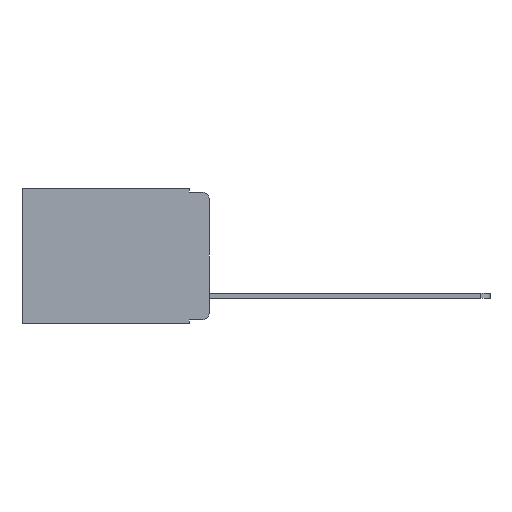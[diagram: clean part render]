
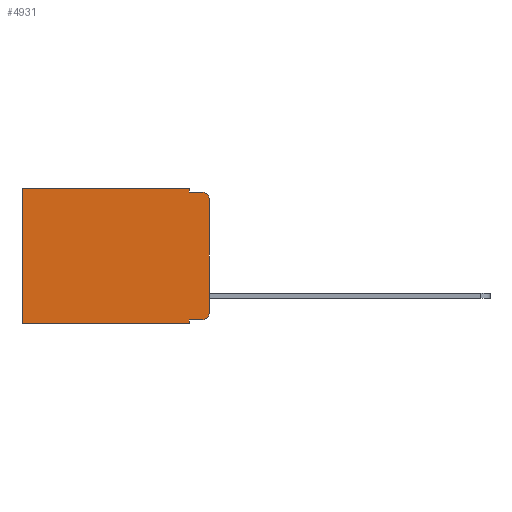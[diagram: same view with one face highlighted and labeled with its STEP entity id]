
A CAD part, left-side view. The second image highlights one B-rep face of the part: STEP entity #4931.
In plain terms, the highlighted planar face has unit normal (-1, 0, 0).
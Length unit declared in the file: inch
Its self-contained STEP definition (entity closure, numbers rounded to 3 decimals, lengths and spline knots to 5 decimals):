
#143 = CARTESIAN_POINT ( 'NONE',  ( 0.298, 0.051, 0. ) ) ;
#381 = DIRECTION ( 'NONE',  ( 0., 1., 0. ) ) ;
#595 = VECTOR ( 'NONE', #5572, 39.37008 ) ;
#621 = CARTESIAN_POINT ( 'NONE',  ( 0.298, 0.473, 0. ) ) ;
#640 = CARTESIAN_POINT ( 'NONE',  ( 0.298, 0.473, 0. ) ) ;
#706 = VERTEX_POINT ( 'NONE', #640 ) ;
#814 = ORIENTED_EDGE ( 'NONE', *, *, #1271, .F. ) ;
#954 = LINE ( 'NONE', #12647, #11044 ) ;
#975 = CARTESIAN_POINT ( 'NONE',  ( 0.298, 0.051, -0.343 ) ) ;
#1271 = EDGE_CURVE ( 'NONE', #1535, #10367, #11282, .T. ) ;
#1535 = VERTEX_POINT ( 'NONE', #975 ) ;
#2124 = LINE ( 'NONE', #621, #5305 ) ;
#2425 = FACE_OUTER_BOUND ( 'NONE', #9493, .T. ) ;
#2588 = ORIENTED_EDGE ( 'NONE', *, *, #4125, .F. ) ;
#2693 = DIRECTION ( 'NONE',  ( -1., 0., 0. ) ) ;
#2719 = VERTEX_POINT ( 'NONE', #5087 ) ;
#2850 = VERTEX_POINT ( 'NONE', #7768 ) ;
#3081 = VERTEX_POINT ( 'NONE', #11312 ) ;
#3576 = DIRECTION ( 'NONE',  ( -1., 0., 0. ) ) ;
#3596 = LINE ( 'NONE', #143, #11508 ) ;
#3645 = CARTESIAN_POINT ( 'NONE',  ( 0.298, 0.473, -0.343 ) ) ;
#3859 = EDGE_CURVE ( 'NONE', #11852, #1535, #12312, .T. ) ;
#3993 = VERTEX_POINT ( 'NONE', #8887 ) ;
#4125 = EDGE_CURVE ( 'NONE', #2850, #7974, #3596, .T. ) ;
#4300 = ORIENTED_EDGE ( 'NONE', *, *, #10126, .T. ) ;
#4311 = EDGE_CURVE ( 'NONE', #11852, #3081, #11987, .T. ) ;
#4498 = ORIENTED_EDGE ( 'NONE', *, *, #12675, .F. ) ;
#4522 = CIRCLE ( 'NONE', #8529, 0.02 ) ;
#4931 = ADVANCED_FACE ( 'NONE', ( #2425 ), #10984, .F. ) ;
#5087 = CARTESIAN_POINT ( 'NONE',  ( 0.298, 0.02, -0.01 ) ) ;
#5145 = DIRECTION ( 'NONE',  ( 1., 0., 0. ) ) ;
#5178 = CARTESIAN_POINT ( 'NONE',  ( 0.298, 0.02, -0.03 ) ) ;
#5304 = ORIENTED_EDGE ( 'NONE', *, *, #4311, .T. ) ;
#5305 = VECTOR ( 'NONE', #8052, 39.37008 ) ;
#5371 = AXIS2_PLACEMENT_3D ( 'NONE', #5178, #3576, #7369 ) ;
#5572 = DIRECTION ( 'NONE',  ( 0., -1., 0. ) ) ;
#5716 = CARTESIAN_POINT ( 'NONE',  ( 0.298, 0., -0.343 ) ) ;
#6243 = CARTESIAN_POINT ( 'NONE',  ( 0.298, 0.051, -0.333 ) ) ;
#6254 = AXIS2_PLACEMENT_3D ( 'NONE', #12766, #5145, #7292 ) ;
#6681 = VECTOR ( 'NONE', #381, 39.37008 ) ;
#6712 = EDGE_CURVE ( 'NONE', #10533, #2719, #10645, .T. ) ;
#6837 = ORIENTED_EDGE ( 'NONE', *, *, #7906, .T. ) ;
#6873 = CARTESIAN_POINT ( 'NONE',  ( 0.298, 0.051, -0.333 ) ) ;
#7198 = CARTESIAN_POINT ( 'NONE',  ( 0.298, 0., -0.03 ) ) ;
#7292 = DIRECTION ( 'NONE',  ( 0., 0., -1. ) ) ;
#7369 = DIRECTION ( 'NONE',  ( 0., 0., -1. ) ) ;
#7660 = ORIENTED_EDGE ( 'NONE', *, *, #11418, .F. ) ;
#7768 = CARTESIAN_POINT ( 'NONE',  ( 0.298, 0.051, 0. ) ) ;
#7906 = EDGE_CURVE ( 'NONE', #3081, #3993, #4522, .T. ) ;
#7974 = VERTEX_POINT ( 'NONE', #8724 ) ;
#8052 = DIRECTION ( 'NONE',  ( 0., 0., -1. ) ) ;
#8434 = DIRECTION ( 'NONE',  ( 0., -1., 0. ) ) ;
#8529 = AXIS2_PLACEMENT_3D ( 'NONE', #8992, #2693, #9982 ) ;
#8589 = ORIENTED_EDGE ( 'NONE', *, *, #11039, .T. ) ;
#8639 = VECTOR ( 'NONE', #11944, 39.37008 ) ;
#8724 = CARTESIAN_POINT ( 'NONE',  ( 0.298, 0.051, -0.01 ) ) ;
#8887 = CARTESIAN_POINT ( 'NONE',  ( 0.298, 0., -0.313 ) ) ;
#8992 = CARTESIAN_POINT ( 'NONE',  ( 0.298, 0.02, -0.313 ) ) ;
#9296 = LINE ( 'NONE', #12703, #595 ) ;
#9307 = VECTOR ( 'NONE', #8434, 39.37008 ) ;
#9329 = CARTESIAN_POINT ( 'NONE',  ( 0.298, 0.051, 0. ) ) ;
#9493 = EDGE_LOOP ( 'NONE', ( #7660, #9689, #4498, #2588, #4300, #8589, #814, #13011, #5304, #6837 ) ) ;
#9524 = CARTESIAN_POINT ( 'NONE',  ( 0.298, 0., 0. ) ) ;
#9637 = VECTOR ( 'NONE', #10303, 39.37008 ) ;
#9689 = ORIENTED_EDGE ( 'NONE', *, *, #6712, .T. ) ;
#9982 = DIRECTION ( 'NONE',  ( 0., 0., -1. ) ) ;
#10126 = EDGE_CURVE ( 'NONE', #2850, #706, #11743, .T. ) ;
#10303 = DIRECTION ( 'NONE',  ( 0., 0., -1. ) ) ;
#10367 = VERTEX_POINT ( 'NONE', #3645 ) ;
#10533 = VERTEX_POINT ( 'NONE', #7198 ) ;
#10635 = DIRECTION ( 'NONE',  ( 0., 0., -1. ) ) ;
#10645 = CIRCLE ( 'NONE', #5371, 0.02 ) ;
#10984 = PLANE ( 'NONE',  #6254 ) ;
#11039 = EDGE_CURVE ( 'NONE', #706, #10367, #2124, .T. ) ;
#11044 = VECTOR ( 'NONE', #10635, 39.37008 ) ;
#11282 = LINE ( 'NONE', #5716, #8639 ) ;
#11312 = CARTESIAN_POINT ( 'NONE',  ( 0.298, 0.02, -0.333 ) ) ;
#11418 = EDGE_CURVE ( 'NONE', #10533, #3993, #954, .T. ) ;
#11508 = VECTOR ( 'NONE', #12392, 39.37008 ) ;
#11743 = LINE ( 'NONE', #9524, #6681 ) ;
#11852 = VERTEX_POINT ( 'NONE', #6243 ) ;
#11944 = DIRECTION ( 'NONE',  ( 0., 1., 0. ) ) ;
#11987 = LINE ( 'NONE', #6873, #9307 ) ;
#12312 = LINE ( 'NONE', #9329, #9637 ) ;
#12392 = DIRECTION ( 'NONE',  ( 0., 0., -1. ) ) ;
#12647 = CARTESIAN_POINT ( 'NONE',  ( 0.298, 0., 0. ) ) ;
#12675 = EDGE_CURVE ( 'NONE', #7974, #2719, #9296, .T. ) ;
#12703 = CARTESIAN_POINT ( 'NONE',  ( 0.298, 0.051, -0.01 ) ) ;
#12766 = CARTESIAN_POINT ( 'NONE',  ( 0.298, 0., 0. ) ) ;
#13011 = ORIENTED_EDGE ( 'NONE', *, *, #3859, .F. ) ;
